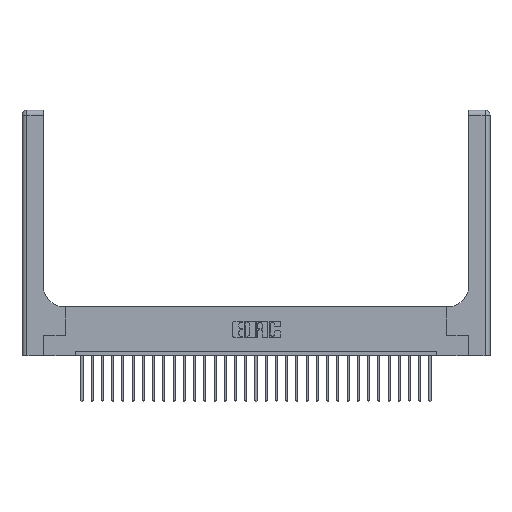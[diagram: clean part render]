
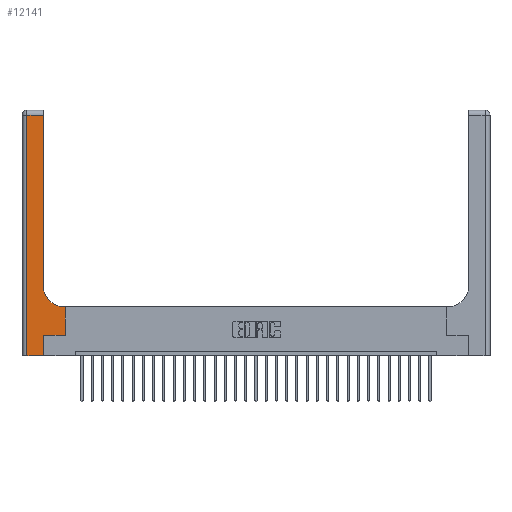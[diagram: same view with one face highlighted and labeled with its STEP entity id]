
A CAD part, top view. The second image highlights one B-rep face of the part: STEP entity #12141.
In plain terms, the highlighted planar face has unit normal (0, 0, 1).
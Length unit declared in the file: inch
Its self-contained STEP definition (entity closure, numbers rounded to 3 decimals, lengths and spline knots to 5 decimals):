
#709 = LINE ( 'NONE', #24191, #7452 ) ;
#1186 = CARTESIAN_POINT ( 'NONE',  ( 0.528, 0.25, 0.37 ) ) ;
#2297 = DIRECTION ( 'NONE',  ( 1., 0., 0. ) ) ;
#2933 = VERTEX_POINT ( 'NONE', #8899 ) ;
#3083 = EDGE_CURVE ( 'NONE', #19541, #15750, #23325, .T. ) ;
#3233 = VERTEX_POINT ( 'NONE', #27754 ) ;
#3426 = DIRECTION ( 'NONE',  ( -1., 0., 0. ) ) ;
#3437 = CARTESIAN_POINT ( 'NONE',  ( 0.265, 0., 0.37 ) ) ;
#3550 = ORIENTED_EDGE ( 'NONE', *, *, #8222, .T. ) ;
#3597 = VECTOR ( 'NONE', #16635, 39.37008 ) ;
#3710 = DIRECTION ( 'NONE',  ( 0., 0., -1. ) ) ;
#3836 = ORIENTED_EDGE ( 'NONE', *, *, #20848, .T. ) ;
#4082 = VECTOR ( 'NONE', #17566, 39.37008 ) ;
#5666 = DIRECTION ( 'NONE',  ( -1., 0., 0. ) ) ;
#5802 = ORIENTED_EDGE ( 'NONE', *, *, #27540, .T. ) ;
#5912 = CARTESIAN_POINT ( 'NONE',  ( 0.51, 0.85, 0.37 ) ) ;
#6420 = CARTESIAN_POINT ( 'NONE',  ( 0.265, 0., 0.37 ) ) ;
#6729 = AXIS2_PLACEMENT_3D ( 'NONE', #5912, #17205, #21219 ) ;
#7143 = ORIENTED_EDGE ( 'NONE', *, *, #21692, .T. ) ;
#7240 = CARTESIAN_POINT ( 'NONE',  ( 0.26, 3., 0.37 ) ) ;
#7370 = LINE ( 'NONE', #1186, #3597 ) ;
#7452 = VECTOR ( 'NONE', #17470, 39.37008 ) ;
#7529 = VECTOR ( 'NONE', #20572, 39.37008 ) ;
#8222 = EDGE_CURVE ( 'NONE', #25815, #27959, #17221, .T. ) ;
#8292 = CARTESIAN_POINT ( 'NONE',  ( 0., 3., 0.37 ) ) ;
#8899 = CARTESIAN_POINT ( 'NONE',  ( 0.528, 0.6, 0.37 ) ) ;
#9268 = VECTOR ( 'NONE', #2297, 39.37008 ) ;
#9520 = CARTESIAN_POINT ( 'NONE',  ( 0.26, 0.85, 0.37 ) ) ;
#9713 = ORIENTED_EDGE ( 'NONE', *, *, #3083, .T. ) ;
#9863 = VERTEX_POINT ( 'NONE', #17895 ) ;
#10111 = CARTESIAN_POINT ( 'NONE',  ( 0.26, 0.6, 0.37 ) ) ;
#10534 = VERTEX_POINT ( 'NONE', #17521 ) ;
#11627 = CARTESIAN_POINT ( 'NONE',  ( 0.51, 0.6, 0.37 ) ) ;
#11829 = ORIENTED_EDGE ( 'NONE', *, *, #25316, .T. ) ;
#11953 = EDGE_LOOP ( 'NONE', ( #11829, #22787, #15133, #23707, #9713, #5802, #3836, #7143, #3550 ) ) ;
#12141 = ADVANCED_FACE ( 'NONE', ( #25459 ), #14439, .F. ) ;
#12405 = EDGE_CURVE ( 'NONE', #25502, #3233, #26752, .T. ) ;
#12841 = LINE ( 'NONE', #16986, #4082 ) ;
#13385 = LINE ( 'NONE', #7240, #17392 ) ;
#14356 = AXIS2_PLACEMENT_3D ( 'NONE', #8292, #3710, #3426 ) ;
#14439 = PLANE ( 'NONE',  #14356 ) ;
#15133 = ORIENTED_EDGE ( 'NONE', *, *, #12405, .T. ) ;
#15737 = LINE ( 'NONE', #15872, #9268 ) ;
#15750 = VERTEX_POINT ( 'NONE', #25245 ) ;
#15872 = CARTESIAN_POINT ( 'NONE',  ( 0.265, 0.25, 0.37 ) ) ;
#16635 = DIRECTION ( 'NONE',  ( 0., 1., 0. ) ) ;
#16986 = CARTESIAN_POINT ( 'NONE',  ( 0., 2.94, 0.37 ) ) ;
#17205 = DIRECTION ( 'NONE',  ( 0., 0., -1. ) ) ;
#17221 = CIRCLE ( 'NONE', #6729, 0.25 ) ;
#17392 = VECTOR ( 'NONE', #22271, 39.37008 ) ;
#17470 = DIRECTION ( 'NONE',  ( 1., 0., 0. ) ) ;
#17521 = CARTESIAN_POINT ( 'NONE',  ( 0.26, 2.94, 0.37 ) ) ;
#17566 = DIRECTION ( 'NONE',  ( -1., 0., 0. ) ) ;
#17895 = CARTESIAN_POINT ( 'NONE',  ( 0.528, 0.25, 0.37 ) ) ;
#19541 = VERTEX_POINT ( 'NONE', #6420 ) ;
#20173 = EDGE_CURVE ( 'NONE', #10534, #25502, #12841, .T. ) ;
#20519 = CARTESIAN_POINT ( 'NONE',  ( 0.06, 2.94, 0.37 ) ) ;
#20572 = DIRECTION ( 'NONE',  ( 0., -1., 0. ) ) ;
#20599 = DIRECTION ( 'NONE',  ( 0., 1., 0. ) ) ;
#20848 = EDGE_CURVE ( 'NONE', #9863, #2933, #7370, .T. ) ;
#21219 = DIRECTION ( 'NONE',  ( 1., 0., 0. ) ) ;
#21692 = EDGE_CURVE ( 'NONE', #2933, #25815, #27141, .T. ) ;
#22271 = DIRECTION ( 'NONE',  ( 0., 1., 0. ) ) ;
#22377 = VECTOR ( 'NONE', #5666, 39.37008 ) ;
#22787 = ORIENTED_EDGE ( 'NONE', *, *, #20173, .T. ) ;
#22896 = VECTOR ( 'NONE', #20599, 39.37008 ) ;
#23013 = CARTESIAN_POINT ( 'NONE',  ( 0.06, 3., 0.37 ) ) ;
#23325 = LINE ( 'NONE', #3437, #22896 ) ;
#23707 = ORIENTED_EDGE ( 'NONE', *, *, #27584, .T. ) ;
#24191 = CARTESIAN_POINT ( 'NONE',  ( 0., 0., 0.37 ) ) ;
#25245 = CARTESIAN_POINT ( 'NONE',  ( 0.265, 0.25, 0.37 ) ) ;
#25316 = EDGE_CURVE ( 'NONE', #27959, #10534, #13385, .T. ) ;
#25459 = FACE_OUTER_BOUND ( 'NONE', #11953, .T. ) ;
#25502 = VERTEX_POINT ( 'NONE', #20519 ) ;
#25815 = VERTEX_POINT ( 'NONE', #11627 ) ;
#26752 = LINE ( 'NONE', #23013, #7529 ) ;
#27141 = LINE ( 'NONE', #10111, #22377 ) ;
#27540 = EDGE_CURVE ( 'NONE', #15750, #9863, #15737, .T. ) ;
#27584 = EDGE_CURVE ( 'NONE', #3233, #19541, #709, .T. ) ;
#27754 = CARTESIAN_POINT ( 'NONE',  ( 0.06, 0., 0.37 ) ) ;
#27959 = VERTEX_POINT ( 'NONE', #9520 ) ;
